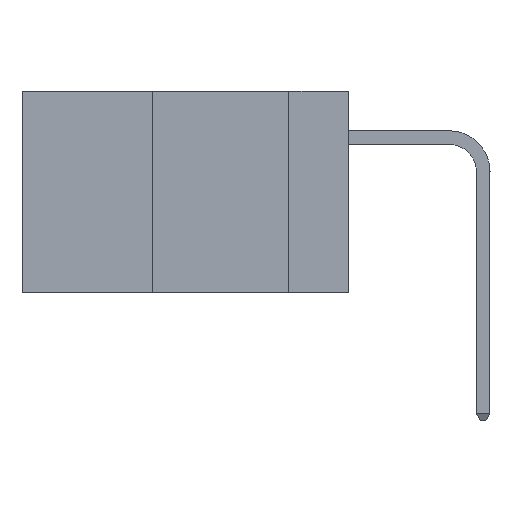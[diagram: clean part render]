
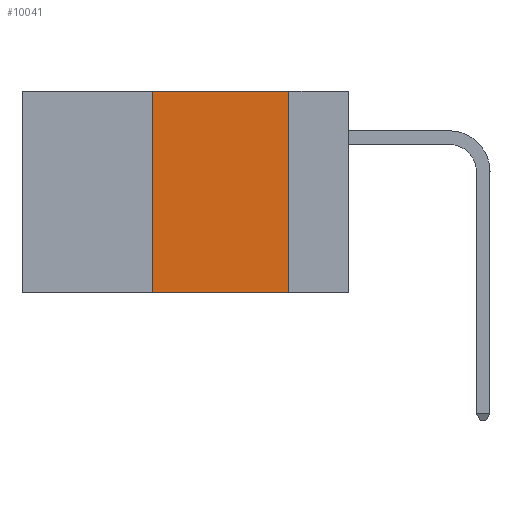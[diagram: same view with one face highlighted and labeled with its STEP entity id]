
A CAD part, left-side view. The second image highlights one B-rep face of the part: STEP entity #10041.
In plain terms, the highlighted planar face has unit normal (-1, 0, 0).
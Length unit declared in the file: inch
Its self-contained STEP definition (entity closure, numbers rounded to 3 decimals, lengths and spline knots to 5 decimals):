
#2057 = CARTESIAN_POINT ( 'NONE',  ( 0., 0.11, -0.37 ) ) ;
#2363 = CARTESIAN_POINT ( 'NONE',  ( 0., 0.36, 0. ) ) ;
#2493 = VERTEX_POINT ( 'NONE', #22061 ) ;
#4993 = LINE ( 'NONE', #8506, #12638 ) ;
#5501 = EDGE_CURVE ( 'NONE', #23395, #33760, #26892, .T. ) ;
#5855 = PLANE ( 'NONE',  #43018 ) ;
#6596 = LINE ( 'NONE', #21468, #25236 ) ;
#6826 = ORIENTED_EDGE ( 'NONE', *, *, #14950, .F. ) ;
#8506 = CARTESIAN_POINT ( 'NONE',  ( 0., 0.36, 0. ) ) ;
#9610 = CARTESIAN_POINT ( 'NONE',  ( 0., 0.11, 0. ) ) ;
#10041 = ADVANCED_FACE ( 'NONE', ( #33918 ), #5855, .F. ) ;
#12239 = LINE ( 'NONE', #9610, #30764 ) ;
#12638 = VECTOR ( 'NONE', #34253, 39.37008 ) ;
#13427 = DIRECTION ( 'NONE',  ( 0., 0., -1. ) ) ;
#14950 = EDGE_CURVE ( 'NONE', #2493, #23395, #4993, .T. ) ;
#16005 = VECTOR ( 'NONE', #45521, 39.37008 ) ;
#17461 = EDGE_CURVE ( 'NONE', #2493, #46555, #6596, .T. ) ;
#21468 = CARTESIAN_POINT ( 'NONE',  ( 0., 0.6, -0.37 ) ) ;
#22061 = CARTESIAN_POINT ( 'NONE',  ( 0., 0.36, -0.37 ) ) ;
#23395 = VERTEX_POINT ( 'NONE', #2363 ) ;
#25236 = VECTOR ( 'NONE', #39700, 39.37008 ) ;
#26892 = LINE ( 'NONE', #27185, #16005 ) ;
#27185 = CARTESIAN_POINT ( 'NONE',  ( 0., 0.6, 0. ) ) ;
#27828 = ORIENTED_EDGE ( 'NONE', *, *, #17461, .T. ) ;
#29089 = CARTESIAN_POINT ( 'NONE',  ( 0., 0.11, 0. ) ) ;
#30764 = VECTOR ( 'NONE', #39114, 39.37008 ) ;
#31547 = ORIENTED_EDGE ( 'NONE', *, *, #40448, .F. ) ;
#31839 = CARTESIAN_POINT ( 'NONE',  ( 0., 0.6, 0. ) ) ;
#33760 = VERTEX_POINT ( 'NONE', #29089 ) ;
#33918 = FACE_OUTER_BOUND ( 'NONE', #38362, .T. ) ;
#34253 = DIRECTION ( 'NONE',  ( 0., 0., 1. ) ) ;
#35455 = DIRECTION ( 'NONE',  ( 1., 0., 0. ) ) ;
#38362 = EDGE_LOOP ( 'NONE', ( #31547, #41814, #6826, #27828 ) ) ;
#39114 = DIRECTION ( 'NONE',  ( 0., 0., -1. ) ) ;
#39700 = DIRECTION ( 'NONE',  ( 0., -1., 0. ) ) ;
#40448 = EDGE_CURVE ( 'NONE', #33760, #46555, #12239, .T. ) ;
#41814 = ORIENTED_EDGE ( 'NONE', *, *, #5501, .F. ) ;
#43018 = AXIS2_PLACEMENT_3D ( 'NONE', #31839, #35455, #13427 ) ;
#45521 = DIRECTION ( 'NONE',  ( 0., -1., 0. ) ) ;
#46555 = VERTEX_POINT ( 'NONE', #2057 ) ;
